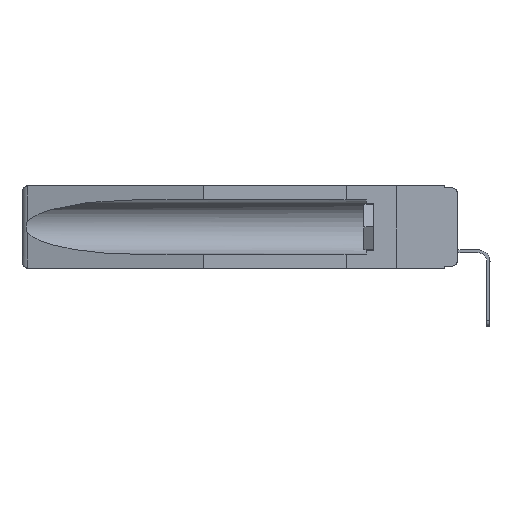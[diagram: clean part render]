
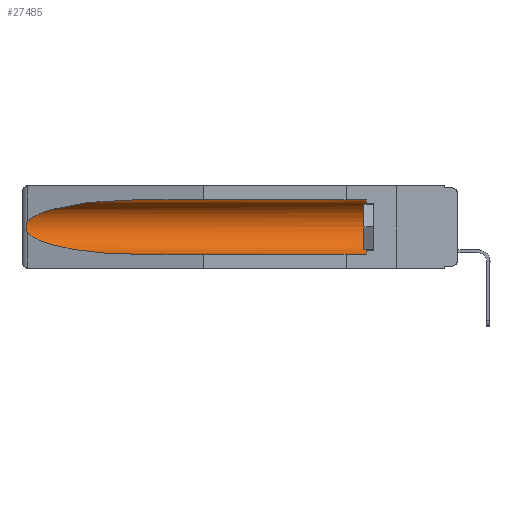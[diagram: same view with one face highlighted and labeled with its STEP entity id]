
A CAD part, left-side view. The second image highlights one B-rep face of the part: STEP entity #27485.
In plain terms, the highlighted cylindrical face has radius 2.857 mm (diameter 5.715 mm), a partial arc.
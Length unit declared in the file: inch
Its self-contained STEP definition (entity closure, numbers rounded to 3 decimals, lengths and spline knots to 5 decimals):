
#163 = CARTESIAN_POINT ( 'NONE',  ( 0.155, 1.07973, -0.284 ) ) ;
#806 = AXIS2_PLACEMENT_3D ( 'NONE', #3353, #24619, #22564 ) ;
#1230 = ORIENTED_EDGE ( 'NONE', *, *, #24123, .T. ) ;
#1415 = ORIENTED_EDGE ( 'NONE', *, *, #18491, .T. ) ;
#2129 = CARTESIAN_POINT ( 'NONE',  ( 0.2673, 1.5327, -0.16383 ) ) ;
#2221 = CARTESIAN_POINT ( 'NONE',  ( 0.26537, 1.52718, -0.19328 ) ) ;
#3353 = CARTESIAN_POINT ( 'NONE',  ( 0.155, -0.30754, -0.1715 ) ) ;
#3440 = CARTESIAN_POINT ( 'NONE',  ( 0.155, -0.30754, -0.284 ) ) ;
#3690 = VECTOR ( 'NONE', #12582, 39.37008 ) ;
#4094 = VERTEX_POINT ( 'NONE', #27129 ) ;
#4185 = CARTESIAN_POINT ( 'NONE',  ( 0.155, 1.07973, -0.059 ) ) ;
#4293 = CARTESIAN_POINT ( 'NONE',  ( 0.26537, 1.52718, -0.14972 ) ) ;
#4539 = CARTESIAN_POINT ( 'NONE',  ( 0.26537, 1.52718, -0.19328 ) ) ;
#5384 = CARTESIAN_POINT ( 'NONE',  ( 0.26537, 1.52718, -0.14972 ) ) ;
#6253 = CARTESIAN_POINT ( 'NONE',  ( 0.26597, 1.52961, -0.15275 ) ) ;
#6347 = VERTEX_POINT ( 'NONE', #18134 ) ;
#6351 = CARTESIAN_POINT ( 'NONE',  ( 0.155, 1.07973, -0.284 ) ) ;
#6697 = LINE ( 'NONE', #3440, #11339 ) ;
#6748 = EDGE_CURVE ( 'NONE', #20069, #4094, #15859, .T. ) ;
#6781 = EDGE_CURVE ( 'NONE', #19504, #6347, #10008, .T. ) ;
#8287 = CARTESIAN_POINT ( 'NONE',  ( 0.155, -0.30754, -0.059 ) ) ;
#8423 = ORIENTED_EDGE ( 'NONE', *, *, #12981, .F. ) ;
#8478 = CARTESIAN_POINT ( 'NONE',  ( 0.2675, 1.53308, -0.17534 ) ) ;
#9686 =( BOUNDED_CURVE ( )  B_SPLINE_CURVE ( 3, ( #4539, #21484, #15420, #163 ),
 .UNSPECIFIED., .F., .F. ) 
 B_SPLINE_CURVE_WITH_KNOTS ( ( 4, 4 ),
 ( 0.1948, 1.5708 ),
 .UNSPECIFIED. ) 
 CURVE ( )  GEOMETRIC_REPRESENTATION_ITEM ( )  RATIONAL_B_SPLINE_CURVE ( ( 1., 0.848, 0.848, 1. ) ) 
 REPRESENTATION_ITEM ( '' )  );
#10008 = LINE ( 'NONE', #8287, #3690 ) ;
#10414 =( BOUNDED_CURVE ( )  B_SPLINE_CURVE ( 3, ( #4185, #12942, #19273, #5384 ),
 .UNSPECIFIED., .F., .F. ) 
 B_SPLINE_CURVE_WITH_KNOTS ( ( 4, 4 ),
 ( 4.71239, 6.08839 ),
 .UNSPECIFIED. ) 
 CURVE ( )  GEOMETRIC_REPRESENTATION_ITEM ( )  RATIONAL_B_SPLINE_CURVE ( ( 1., 0.848, 0.848, 1. ) ) 
 REPRESENTATION_ITEM ( '' )  );
#10554 = CARTESIAN_POINT ( 'NONE',  ( 0.155, 0.126, -0.284 ) ) ;
#11339 = VECTOR ( 'NONE', #22649, 39.37008 ) ;
#12582 = DIRECTION ( 'NONE',  ( 0., 1., 0. ) ) ;
#12942 = CARTESIAN_POINT ( 'NONE',  ( 0.21114, 1.30732, -0.059 ) ) ;
#12981 = EDGE_CURVE ( 'NONE', #17602, #19858, #6697, .T. ) ;
#14138 = CYLINDRICAL_SURFACE ( 'NONE', #806, 0.1125 ) ;
#14812 = CARTESIAN_POINT ( 'NONE',  ( 0.26654, 1.53092, -0.15636 ) ) ;
#15000 = CARTESIAN_POINT ( 'NONE',  ( 0.26597, 1.5296, -0.19026 ) ) ;
#15420 = CARTESIAN_POINT ( 'NONE',  ( 0.21114, 1.30732, -0.284 ) ) ;
#15495 = EDGE_CURVE ( 'NONE', #4094, #19858, #9686, .T. ) ;
#15630 = CARTESIAN_POINT ( 'NONE',  ( 0.26537, 1.52718, -0.14972 ) ) ;
#15859 = B_SPLINE_CURVE_WITH_KNOTS ( 'NONE', 3,
 ( #4293, #6253, #14812, #2129, #18839, #8478, #23304, #25559, #15000, #2221 ),
 .UNSPECIFIED., .F., .F.,
 ( 4, 2, 2, 2, 4 ),
 ( 0., 0.00029, 0.00058, 0.00087, 0.00117 ),
 .UNSPECIFIED. ) ;
#16466 = DIRECTION ( 'NONE',  ( 0., 0., 1. ) ) ;
#16647 = CARTESIAN_POINT ( 'NONE',  ( 0.155, 0.126, -0.1715 ) ) ;
#17148 = CIRCLE ( 'NONE', #20005, 0.1125 ) ;
#17469 = ORIENTED_EDGE ( 'NONE', *, *, #6748, .T. ) ;
#17515 = CARTESIAN_POINT ( 'NONE',  ( 0.155, 0.126, -0.059 ) ) ;
#17602 = VERTEX_POINT ( 'NONE', #10554 ) ;
#18134 = CARTESIAN_POINT ( 'NONE',  ( 0.155, 1.07973, -0.059 ) ) ;
#18425 = FACE_OUTER_BOUND ( 'NONE', #19156, .T. ) ;
#18491 = EDGE_CURVE ( 'NONE', #17602, #19504, #17148, .T. ) ;
#18819 = DIRECTION ( 'NONE',  ( 0., -1., 0. ) ) ;
#18839 = CARTESIAN_POINT ( 'NONE',  ( 0.2675, 1.53308, -0.16763 ) ) ;
#19156 = EDGE_LOOP ( 'NONE', ( #1230, #17469, #19788, #8423, #1415, #20867 ) ) ;
#19273 = CARTESIAN_POINT ( 'NONE',  ( 0.25451, 1.48313, -0.09465 ) ) ;
#19504 = VERTEX_POINT ( 'NONE', #17515 ) ;
#19788 = ORIENTED_EDGE ( 'NONE', *, *, #15495, .T. ) ;
#19858 = VERTEX_POINT ( 'NONE', #6351 ) ;
#20005 = AXIS2_PLACEMENT_3D ( 'NONE', #16647, #18819, #16466 ) ;
#20069 = VERTEX_POINT ( 'NONE', #15630 ) ;
#20867 = ORIENTED_EDGE ( 'NONE', *, *, #6781, .T. ) ;
#21484 = CARTESIAN_POINT ( 'NONE',  ( 0.25451, 1.48313, -0.24835 ) ) ;
#22564 = DIRECTION ( 'NONE',  ( 0., 0., 1. ) ) ;
#22649 = DIRECTION ( 'NONE',  ( 0., 1., 0. ) ) ;
#23304 = CARTESIAN_POINT ( 'NONE',  ( 0.2673, 1.53269, -0.17917 ) ) ;
#24123 = EDGE_CURVE ( 'NONE', #6347, #20069, #10414, .T. ) ;
#24619 = DIRECTION ( 'NONE',  ( 0., 1., 0. ) ) ;
#25559 = CARTESIAN_POINT ( 'NONE',  ( 0.26655, 1.53094, -0.18657 ) ) ;
#27129 = CARTESIAN_POINT ( 'NONE',  ( 0.26537, 1.52718, -0.19328 ) ) ;
#27485 = ADVANCED_FACE ( 'NONE', ( #18425 ), #14138, .F. ) ;
